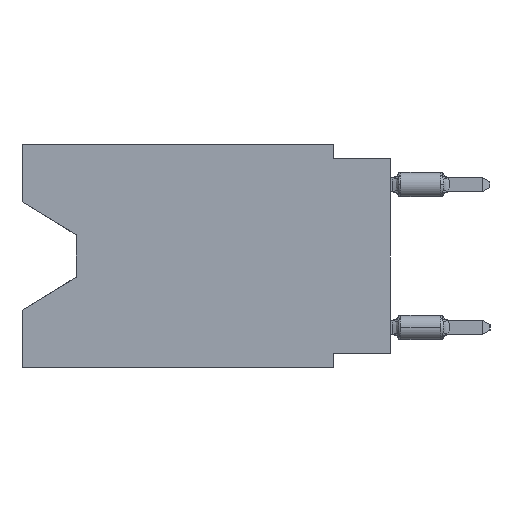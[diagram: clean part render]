
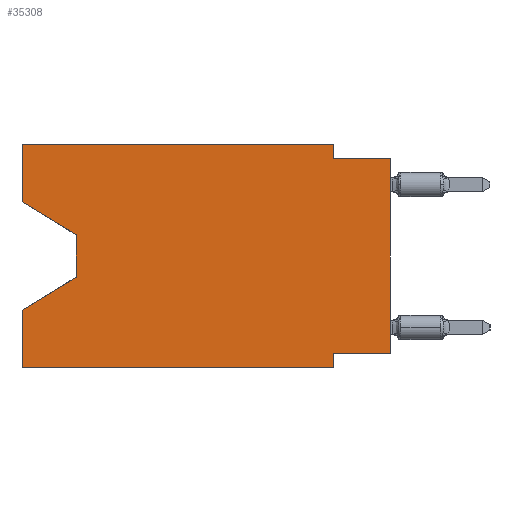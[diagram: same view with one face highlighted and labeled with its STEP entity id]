
A CAD part, left-side view. The second image highlights one B-rep face of the part: STEP entity #35308.
In plain terms, the highlighted planar face has unit normal (-1, 0, 0).
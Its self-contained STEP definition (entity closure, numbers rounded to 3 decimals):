
#413 = FACE_OUTER_BOUND ( 'NONE', #19540, .T. ) ;
#594 = EDGE_CURVE ( 'NONE', #20841, #12002, #10575, .T. ) ;
#937 = EDGE_CURVE ( 'NONE', #6659, #25869, #28627, .T. ) ;
#941 = DIRECTION ( 'NONE',  ( 0., 0., -1. ) ) ;
#1014 = CARTESIAN_POINT ( 'NONE',  ( 0., 13.97, -5.893 ) ) ;
#1133 = CARTESIAN_POINT ( 'NONE',  ( 0., 16.383, 0. ) ) ;
#1153 = LINE ( 'NONE', #17322, #9665 ) ;
#1186 = CARTESIAN_POINT ( 'NONE',  ( 0., 0., 0. ) ) ;
#1551 = ORIENTED_EDGE ( 'NONE', *, *, #33004, .T. ) ;
#1560 = DIRECTION ( 'NONE',  ( 0., -1., 0. ) ) ;
#2090 = ORIENTED_EDGE ( 'NONE', *, *, #21093, .T. ) ;
#2121 = DIRECTION ( 'NONE',  ( 0., -1., 0. ) ) ;
#2136 = EDGE_CURVE ( 'NONE', #16260, #27964, #28205, .T. ) ;
#2325 = VECTOR ( 'NONE', #18678, 1000. ) ;
#2345 = ORIENTED_EDGE ( 'NONE', *, *, #5863, .F. ) ;
#4109 = CARTESIAN_POINT ( 'NONE',  ( 0., 16.383, 0. ) ) ;
#4385 = VECTOR ( 'NONE', #22994, 1000. ) ;
#4722 = VECTOR ( 'NONE', #15210, 1000. ) ;
#5122 = VECTOR ( 'NONE', #1560, 1000. ) ;
#5166 = CARTESIAN_POINT ( 'NONE',  ( 0., 2.54, -9.271 ) ) ;
#5664 = DIRECTION ( 'NONE',  ( 0., 0., -1. ) ) ;
#5863 = EDGE_CURVE ( 'NONE', #16260, #34592, #12708, .T. ) ;
#5934 = ORIENTED_EDGE ( 'NONE', *, *, #594, .T. ) ;
#6263 = VERTEX_POINT ( 'NONE', #8567 ) ;
#6467 = VECTOR ( 'NONE', #8517, 1000. ) ;
#6516 = DIRECTION ( 'NONE',  ( 1., 0., 0. ) ) ;
#6586 = EDGE_CURVE ( 'NONE', #27964, #20819, #33023, .T. ) ;
#6659 = VERTEX_POINT ( 'NONE', #14774 ) ;
#6757 = CARTESIAN_POINT ( 'NONE',  ( 0., 16.383, -9.906 ) ) ;
#7733 = CARTESIAN_POINT ( 'NONE',  ( 0., 16.383, 0. ) ) ;
#8517 = DIRECTION ( 'NONE',  ( 0., 0., -1. ) ) ;
#8567 = CARTESIAN_POINT ( 'NONE',  ( 0., 16.383, -7.36 ) ) ;
#8950 = VECTOR ( 'NONE', #14873, 1000. ) ;
#9157 = EDGE_CURVE ( 'NONE', #20841, #6263, #9481, .T. ) ;
#9481 = LINE ( 'NONE', #4109, #4722 ) ;
#9665 = VECTOR ( 'NONE', #20162, 1000. ) ;
#9740 = CARTESIAN_POINT ( 'NONE',  ( 0., 16.383, -2.546 ) ) ;
#10384 = AXIS2_PLACEMENT_3D ( 'NONE', #1133, #6516, #941 ) ;
#10575 = LINE ( 'NONE', #27040, #18634 ) ;
#11576 = CARTESIAN_POINT ( 'NONE',  ( 0., 16.383, -2.546 ) ) ;
#11846 = ORIENTED_EDGE ( 'NONE', *, *, #2136, .T. ) ;
#12002 = VERTEX_POINT ( 'NONE', #12135 ) ;
#12135 = CARTESIAN_POINT ( 'NONE',  ( 0., 2.54, -9.906 ) ) ;
#12309 = VERTEX_POINT ( 'NONE', #22816 ) ;
#12315 = LINE ( 'NONE', #1186, #27323 ) ;
#12380 = CARTESIAN_POINT ( 'NONE',  ( 0., 16.383, 0. ) ) ;
#12708 = LINE ( 'NONE', #23765, #28533 ) ;
#14600 = CARTESIAN_POINT ( 'NONE',  ( 0., 13.97, -4.013 ) ) ;
#14774 = CARTESIAN_POINT ( 'NONE',  ( 0., 0., -9.271 ) ) ;
#14872 = EDGE_CURVE ( 'NONE', #20648, #31994, #34524, .T. ) ;
#14873 = DIRECTION ( 'NONE',  ( 0., 1., 0. ) ) ;
#15007 = ORIENTED_EDGE ( 'NONE', *, *, #14872, .F. ) ;
#15210 = DIRECTION ( 'NONE',  ( 0., 0., 1. ) ) ;
#15734 = CARTESIAN_POINT ( 'NONE',  ( 0., 0., -0.635 ) ) ;
#16050 = DIRECTION ( 'NONE',  ( 0., 0.855, -0.519 ) ) ;
#16260 = VERTEX_POINT ( 'NONE', #9740 ) ;
#16417 = EDGE_CURVE ( 'NONE', #34592, #12309, #32251, .T. ) ;
#16589 = LINE ( 'NONE', #19265, #35342 ) ;
#16699 = DIRECTION ( 'NONE',  ( 0., 0., 1. ) ) ;
#17322 = CARTESIAN_POINT ( 'NONE',  ( 0., 2.54, -9.906 ) ) ;
#17394 = ORIENTED_EDGE ( 'NONE', *, *, #6586, .T. ) ;
#17541 = CARTESIAN_POINT ( 'NONE',  ( 0., 0., -9.271 ) ) ;
#18634 = VECTOR ( 'NONE', #2121, 1000. ) ;
#18678 = DIRECTION ( 'NONE',  ( 0., -1., 0. ) ) ;
#19139 = EDGE_CURVE ( 'NONE', #25869, #12002, #1153, .T. ) ;
#19248 = CARTESIAN_POINT ( 'NONE',  ( 0., 13.97, -4.013 ) ) ;
#19265 = CARTESIAN_POINT ( 'NONE',  ( 0., 13.97, -5.893 ) ) ;
#19284 = LINE ( 'NONE', #30179, #23410 ) ;
#19540 = EDGE_LOOP ( 'NONE', ( #11846, #17394, #1551, #25597, #5934, #25104, #27400, #2090, #15007, #23909, #20418, #2345 ) ) ;
#20162 = DIRECTION ( 'NONE',  ( 0., 0., -1. ) ) ;
#20418 = ORIENTED_EDGE ( 'NONE', *, *, #16417, .F. ) ;
#20574 = DIRECTION ( 'NONE',  ( 0., 0., 1. ) ) ;
#20648 = VERTEX_POINT ( 'NONE', #27385 ) ;
#20819 = VERTEX_POINT ( 'NONE', #1014 ) ;
#20841 = VERTEX_POINT ( 'NONE', #6757 ) ;
#21093 = EDGE_CURVE ( 'NONE', #6659, #31994, #12315, .T. ) ;
#21313 = CARTESIAN_POINT ( 'NONE',  ( 0., 0., -0.635 ) ) ;
#22816 = CARTESIAN_POINT ( 'NONE',  ( 0., 2.54, 0. ) ) ;
#22954 = EDGE_CURVE ( 'NONE', #12309, #20648, #19284, .T. ) ;
#22994 = DIRECTION ( 'NONE',  ( 0., -0.855, -0.519 ) ) ;
#23410 = VECTOR ( 'NONE', #5664, 1000. ) ;
#23765 = CARTESIAN_POINT ( 'NONE',  ( 0., 16.383, 0. ) ) ;
#23909 = ORIENTED_EDGE ( 'NONE', *, *, #22954, .F. ) ;
#25104 = ORIENTED_EDGE ( 'NONE', *, *, #19139, .F. ) ;
#25482 = PLANE ( 'NONE',  #10384 ) ;
#25597 = ORIENTED_EDGE ( 'NONE', *, *, #9157, .F. ) ;
#25869 = VERTEX_POINT ( 'NONE', #5166 ) ;
#27040 = CARTESIAN_POINT ( 'NONE',  ( 0., 16.383, -9.906 ) ) ;
#27323 = VECTOR ( 'NONE', #16699, 1000. ) ;
#27385 = CARTESIAN_POINT ( 'NONE',  ( 0., 2.54, -0.635 ) ) ;
#27400 = ORIENTED_EDGE ( 'NONE', *, *, #937, .F. ) ;
#27964 = VERTEX_POINT ( 'NONE', #19248 ) ;
#28205 = LINE ( 'NONE', #11576, #4385 ) ;
#28533 = VECTOR ( 'NONE', #20574, 1000. ) ;
#28627 = LINE ( 'NONE', #17541, #8950 ) ;
#30179 = CARTESIAN_POINT ( 'NONE',  ( 0., 2.54, 0. ) ) ;
#31994 = VERTEX_POINT ( 'NONE', #21313 ) ;
#32251 = LINE ( 'NONE', #7733, #2325 ) ;
#33004 = EDGE_CURVE ( 'NONE', #20819, #6263, #16589, .T. ) ;
#33023 = LINE ( 'NONE', #14600, #6467 ) ;
#34524 = LINE ( 'NONE', #15734, #5122 ) ;
#34592 = VERTEX_POINT ( 'NONE', #12380 ) ;
#35308 = ADVANCED_FACE ( 'NONE', ( #413 ), #25482, .F. ) ;
#35342 = VECTOR ( 'NONE', #16050, 1000. ) ;
